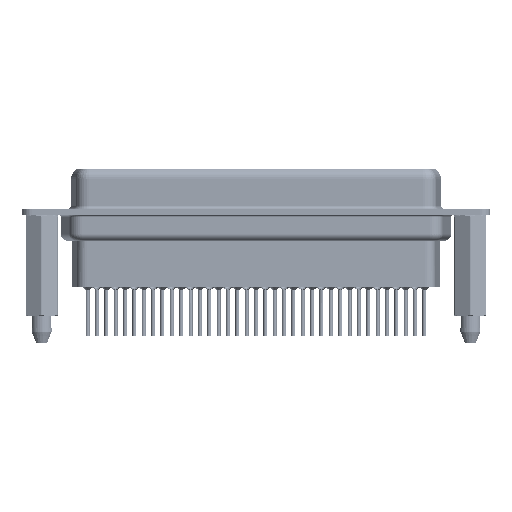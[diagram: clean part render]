
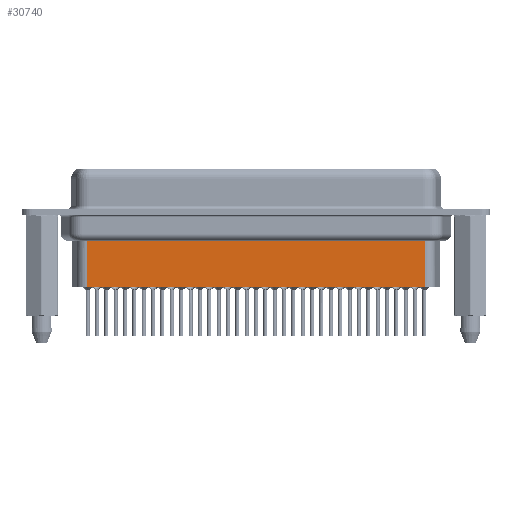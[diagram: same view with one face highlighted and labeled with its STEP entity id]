
A CAD part, front view. The second image highlights one B-rep face of the part: STEP entity #30740.
In plain terms, the highlighted planar face has unit normal (0, -1, 0).
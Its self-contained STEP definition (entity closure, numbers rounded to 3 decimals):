
#618 = VERTEX_POINT ( 'NONE', #11077 ) ;
#641 = CARTESIAN_POINT ( 'NONE',  ( 6.706, -3.5, -3.1 ) ) ;
#1630 = LINE ( 'NONE', #22834, #8952 ) ;
#1782 = DIRECTION ( 'NONE',  ( -1., 0., 0. ) ) ;
#2628 = VECTOR ( 'NONE', #29693, 1000. ) ;
#2724 = EDGE_CURVE ( 'NONE', #19235, #10663, #3678, .T. ) ;
#2939 = ORIENTED_EDGE ( 'NONE', *, *, #2724, .F. ) ;
#3678 = LINE ( 'NONE', #16846, #2628 ) ;
#4338 = CARTESIAN_POINT ( 'NONE',  ( 6.706, -3.5, -11.15 ) ) ;
#6086 = VERTEX_POINT ( 'NONE', #12320 ) ;
#8952 = VECTOR ( 'NONE', #9805, 1000. ) ;
#9805 = DIRECTION ( 'NONE',  ( -1., 0., 0. ) ) ;
#10663 = VERTEX_POINT ( 'NONE', #20570 ) ;
#10666 = DIRECTION ( 'NONE',  ( 0., -1., 0. ) ) ;
#11077 = CARTESIAN_POINT ( 'NONE',  ( 6.706, -3.5, -4.097 ) ) ;
#12320 = CARTESIAN_POINT ( 'NONE',  ( 6.706, -3.5, -11.15 ) ) ;
#15510 = CARTESIAN_POINT ( 'NONE',  ( 56.794, -3.5, -4.097 ) ) ;
#16339 = EDGE_CURVE ( 'NONE', #10663, #6086, #27277, .T. ) ;
#16548 = DIRECTION ( 'NONE',  ( 0., 0., -1. ) ) ;
#16846 = CARTESIAN_POINT ( 'NONE',  ( 56.794, -3.5, -3.1 ) ) ;
#19039 = ORIENTED_EDGE ( 'NONE', *, *, #29061, .T. ) ;
#19077 = FACE_OUTER_BOUND ( 'NONE', #24233, .T. ) ;
#19235 = VERTEX_POINT ( 'NONE', #15510 ) ;
#20570 = CARTESIAN_POINT ( 'NONE',  ( 56.794, -3.5, -11.15 ) ) ;
#21015 = LINE ( 'NONE', #641, #25131 ) ;
#22193 = EDGE_CURVE ( 'NONE', #19235, #618, #1630, .T. ) ;
#22834 = CARTESIAN_POINT ( 'NONE',  ( 6.459, -3.5, -4.097 ) ) ;
#23355 = ORIENTED_EDGE ( 'NONE', *, *, #16339, .F. ) ;
#24233 = EDGE_LOOP ( 'NONE', ( #2939, #30286, #19039, #23355 ) ) ;
#24356 = PLANE ( 'NONE',  #25732 ) ;
#25131 = VECTOR ( 'NONE', #16548, 1000. ) ;
#25732 = AXIS2_PLACEMENT_3D ( 'NONE', #29501, #10666, #26248 ) ;
#26248 = DIRECTION ( 'NONE',  ( 1., 0., 0. ) ) ;
#27277 = LINE ( 'NONE', #4338, #29800 ) ;
#29061 = EDGE_CURVE ( 'NONE', #618, #6086, #21015, .T. ) ;
#29501 = CARTESIAN_POINT ( 'NONE',  ( 6.706, -3.5, -3.1 ) ) ;
#29693 = DIRECTION ( 'NONE',  ( 0., 0., -1. ) ) ;
#29800 = VECTOR ( 'NONE', #1782, 1000. ) ;
#30286 = ORIENTED_EDGE ( 'NONE', *, *, #22193, .T. ) ;
#30740 = ADVANCED_FACE ( 'NONE', ( #19077 ), #24356, .T. ) ;
